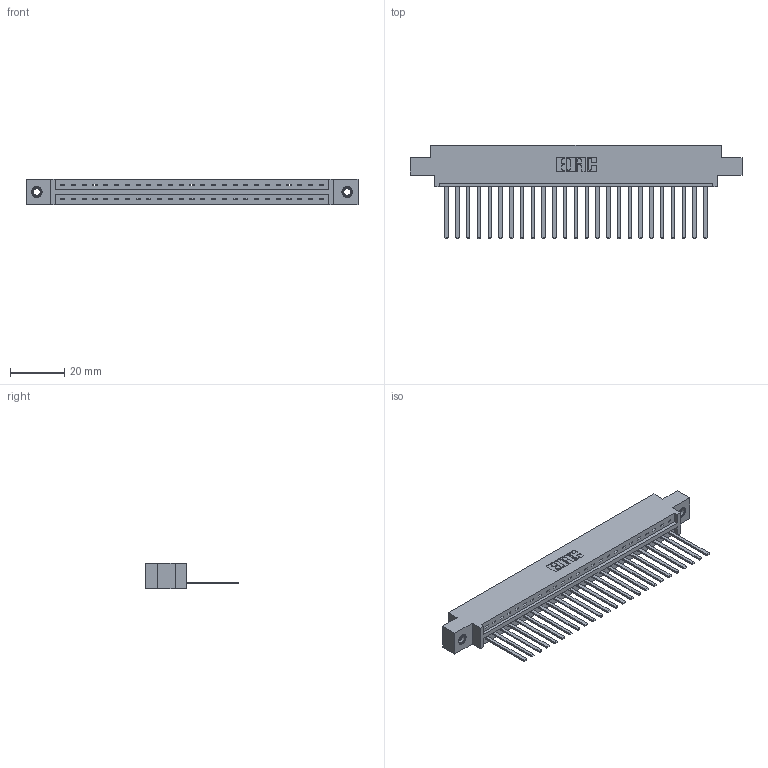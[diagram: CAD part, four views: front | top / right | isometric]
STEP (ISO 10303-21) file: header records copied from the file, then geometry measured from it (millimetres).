
FILE_DESCRIPTION (( 'STEP AP203' ), '1' );
FILE_NAME ('387-025-544-607.STEP', '2019-10-03T12:03:03', ( '' ), ( '' ), 'SwSTEP 2.0', 'SolidWorks 2016', '' );
FILE_SCHEMA (( 'CONFIG_CONTROL_DESIGN' ));
Length unit declared in the file: inch
Products named in the file (4): 337 Part_0.170 Offset - 0.156 Dia-TI; 387-025-544-607; 345-292-001_345-293-144; 345-250-001_345-250-005-103
Assembly tree (28 placements, depth 2):
  387-025-544-607
    337 Part_0.170 Offset - 0.156 Dia-TI
    345-292-001_345-293-144  x25
    345-250-001_345-250-005-103  x2
Bounding box: 122.07 x 34.3 x 9.4 mm (x, y, z)
Volume: 12633.1 mm3; surface area: 14050.1 mm2
Topology: 28 solids, 28 shells, 1578 faces, 4709 edges, 3098 vertices
Faces by surface type: plane 1156, cylinder 406, cone 12, torus 4
Entity records: 21916 total; most frequent: CARTESIAN_POINT 3796, ORIENTED_EDGE 3750, DIRECTION 3259, EDGE_CURVE 1875, VECTOR 1731, LINE 1731, VERTEX_POINT 1244, AXIS2_PLACEMENT_3D 764
